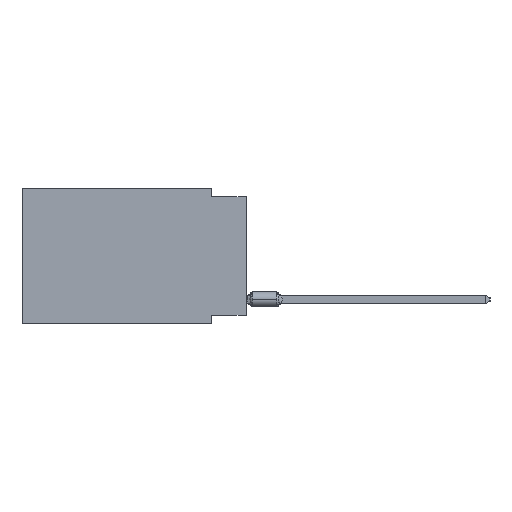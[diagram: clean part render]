
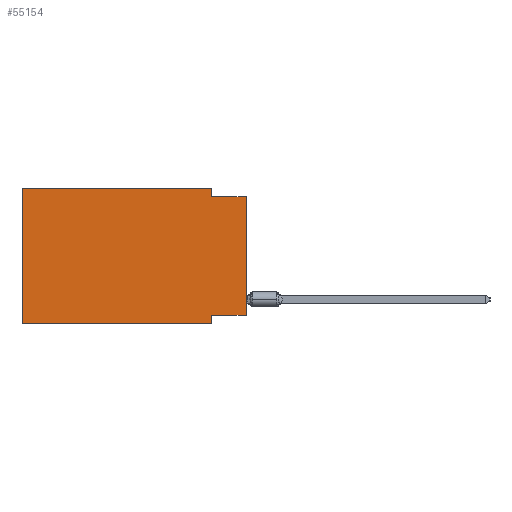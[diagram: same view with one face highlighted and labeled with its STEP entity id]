
A CAD part, left-side view. The second image highlights one B-rep face of the part: STEP entity #55154.
In plain terms, the highlighted planar face has unit normal (-1, 0, 0).
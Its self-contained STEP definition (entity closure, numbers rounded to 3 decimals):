
#789 = EDGE_CURVE ( 'NONE', #54497, #3029, #19694, .T. ) ;
#1155 = CARTESIAN_POINT ( 'NONE',  ( 0., 16.383, 0. ) ) ;
#3029 = VERTEX_POINT ( 'NONE', #1155 ) ;
#3423 = VECTOR ( 'NONE', #60225, 1000. ) ;
#4381 = EDGE_CURVE ( 'NONE', #58455, #9565, #63736, .T. ) ;
#5554 = CARTESIAN_POINT ( 'NONE',  ( 0., 2.54, -9.271 ) ) ;
#5747 = VERTEX_POINT ( 'NONE', #33611 ) ;
#6940 = VERTEX_POINT ( 'NONE', #7069 ) ;
#7069 = CARTESIAN_POINT ( 'NONE',  ( 0., 2.54, 0. ) ) ;
#8510 = ORIENTED_EDGE ( 'NONE', *, *, #23289, .F. ) ;
#8586 = CARTESIAN_POINT ( 'NONE',  ( 0., 16.383, 0. ) ) ;
#9565 = VERTEX_POINT ( 'NONE', #5554 ) ;
#10256 = DIRECTION ( 'NONE',  ( 0., 0., -1. ) ) ;
#10317 = EDGE_CURVE ( 'NONE', #58455, #61911, #15231, .T. ) ;
#10781 = VECTOR ( 'NONE', #10256, 1000. ) ;
#12131 = ORIENTED_EDGE ( 'NONE', *, *, #10317, .T. ) ;
#14544 = DIRECTION ( 'NONE',  ( 0., -1., 0. ) ) ;
#14693 = LINE ( 'NONE', #34687, #33390 ) ;
#15231 = LINE ( 'NONE', #39842, #29694 ) ;
#16198 = DIRECTION ( 'NONE',  ( 0., 0., 1. ) ) ;
#19694 = LINE ( 'NONE', #59388, #56168 ) ;
#20464 = EDGE_CURVE ( 'NONE', #6940, #5747, #60758, .T. ) ;
#20847 = CARTESIAN_POINT ( 'NONE',  ( 0., 16.383, -9.906 ) ) ;
#20985 = DIRECTION ( 'NONE',  ( 0., 0., 1. ) ) ;
#22729 = ORIENTED_EDGE ( 'NONE', *, *, #789, .F. ) ;
#23169 = ORIENTED_EDGE ( 'NONE', *, *, #4381, .F. ) ;
#23289 = EDGE_CURVE ( 'NONE', #3029, #6940, #45394, .T. ) ;
#23658 = PLANE ( 'NONE',  #51233 ) ;
#23784 = VECTOR ( 'NONE', #32934, 1000. ) ;
#24714 = CARTESIAN_POINT ( 'NONE',  ( 0., 16.383, 0. ) ) ;
#24901 = CARTESIAN_POINT ( 'NONE',  ( 0., 0., -9.271 ) ) ;
#25158 = EDGE_CURVE ( 'NONE', #54497, #58384, #30695, .T. ) ;
#29694 = VECTOR ( 'NONE', #16198, 1000. ) ;
#30050 = CARTESIAN_POINT ( 'NONE',  ( 0., 16.383, -9.906 ) ) ;
#30695 = LINE ( 'NONE', #20847, #3423 ) ;
#32243 = EDGE_CURVE ( 'NONE', #9565, #58384, #14693, .T. ) ;
#32643 = VECTOR ( 'NONE', #14544, 1000. ) ;
#32934 = DIRECTION ( 'NONE',  ( 0., -1., 0. ) ) ;
#33110 = CARTESIAN_POINT ( 'NONE',  ( 0., 2.54, -9.906 ) ) ;
#33390 = VECTOR ( 'NONE', #54696, 1000. ) ;
#33611 = CARTESIAN_POINT ( 'NONE',  ( 0., 2.54, -0.635 ) ) ;
#34151 = DIRECTION ( 'NONE',  ( 1., 0., 0. ) ) ;
#34687 = CARTESIAN_POINT ( 'NONE',  ( 0., 2.54, -9.906 ) ) ;
#36441 = VECTOR ( 'NONE', #47395, 1000. ) ;
#37792 = FACE_OUTER_BOUND ( 'NONE', #55418, .T. ) ;
#39842 = CARTESIAN_POINT ( 'NONE',  ( 0., 0., 0. ) ) ;
#41081 = CARTESIAN_POINT ( 'NONE',  ( 0., 2.54, 0. ) ) ;
#45394 = LINE ( 'NONE', #24714, #32643 ) ;
#47395 = DIRECTION ( 'NONE',  ( 0., 1., 0. ) ) ;
#47713 = CARTESIAN_POINT ( 'NONE',  ( 0., 0., -9.271 ) ) ;
#48036 = CARTESIAN_POINT ( 'NONE',  ( 0., 0., -0.635 ) ) ;
#48483 = ORIENTED_EDGE ( 'NONE', *, *, #53473, .F. ) ;
#48890 = ORIENTED_EDGE ( 'NONE', *, *, #20464, .F. ) ;
#49806 = ORIENTED_EDGE ( 'NONE', *, *, #32243, .F. ) ;
#51233 = AXIS2_PLACEMENT_3D ( 'NONE', #8586, #34151, #63349 ) ;
#53473 = EDGE_CURVE ( 'NONE', #5747, #61911, #60058, .T. ) ;
#53513 = CARTESIAN_POINT ( 'NONE',  ( 0., 0., -0.635 ) ) ;
#54497 = VERTEX_POINT ( 'NONE', #30050 ) ;
#54696 = DIRECTION ( 'NONE',  ( 0., 0., -1. ) ) ;
#55154 = ADVANCED_FACE ( 'NONE', ( #37792 ), #23658, .F. ) ;
#55418 = EDGE_LOOP ( 'NONE', ( #12131, #48483, #48890, #8510, #22729, #57245, #49806, #23169 ) ) ;
#56168 = VECTOR ( 'NONE', #20985, 1000. ) ;
#57245 = ORIENTED_EDGE ( 'NONE', *, *, #25158, .T. ) ;
#58384 = VERTEX_POINT ( 'NONE', #33110 ) ;
#58455 = VERTEX_POINT ( 'NONE', #24901 ) ;
#59388 = CARTESIAN_POINT ( 'NONE',  ( 0., 16.383, 0. ) ) ;
#60058 = LINE ( 'NONE', #48036, #23784 ) ;
#60225 = DIRECTION ( 'NONE',  ( 0., -1., 0. ) ) ;
#60758 = LINE ( 'NONE', #41081, #10781 ) ;
#61911 = VERTEX_POINT ( 'NONE', #53513 ) ;
#63349 = DIRECTION ( 'NONE',  ( 0., 0., -1. ) ) ;
#63736 = LINE ( 'NONE', #47713, #36441 ) ;
